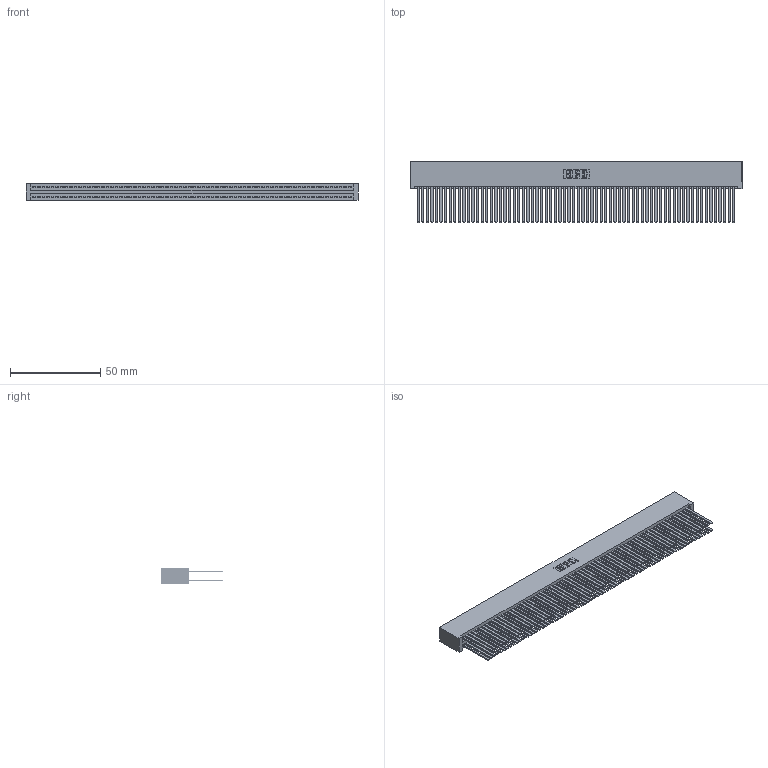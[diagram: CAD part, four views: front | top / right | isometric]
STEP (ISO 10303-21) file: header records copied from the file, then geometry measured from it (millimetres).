
FILE_DESCRIPTION (( 'STEP AP203' ), '1' );
FILE_NAME ('395-140-544-201.STEP', '2018-12-05T22:16:34', ( '' ), ( '' ), 'SwSTEP 2.0', 'SolidWorks 2016', '' );
FILE_SCHEMA (( 'CONFIG_CONTROL_DESIGN' ));
Length unit declared in the file: inch
Products named in the file (3): 345 Part_No Mounting Lugs; 345-292-001_345-293-144; 395-140-544-201
Assembly tree (141 placements, depth 2):
  395-140-544-201
    345 Part_No Mounting Lugs
    345-292-001_345-293-144  x140
Bounding box: 184.4 x 33.96 x 9.4 mm (x, y, z)
Volume: 20751.5 mm3; surface area: 37271.9 mm2
Topology: 141 solids, 141 shells, 6278 faces, 18657 edges, 12250 vertices
Faces by surface type: plane 4136, cylinder 2142
Entity records: 50693 total; most frequent: CARTESIAN_POINT 8468, ORIENTED_EDGE 8402, DIRECTION 7425, EDGE_CURVE 4201, LINE 3801, VECTOR 3801, VERTEX_POINT 2798, AXIS2_PLACEMENT_3D 1812
